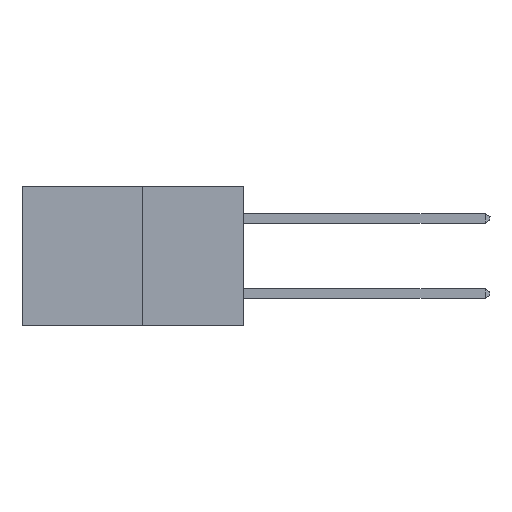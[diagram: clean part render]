
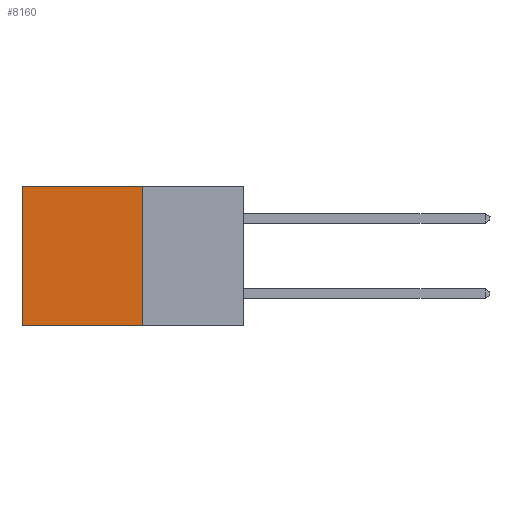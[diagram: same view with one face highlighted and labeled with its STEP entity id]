
A CAD part, left-side view. The second image highlights one B-rep face of the part: STEP entity #8160.
In plain terms, the highlighted planar face has unit normal (-1, 0, 0).
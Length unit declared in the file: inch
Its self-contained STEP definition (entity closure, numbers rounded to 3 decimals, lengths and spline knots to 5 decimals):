
#1149 = EDGE_CURVE ( 'NONE', #7648, #6884, #10491, .T. ) ;
#1304 = FACE_OUTER_BOUND ( 'NONE', #7116, .T. ) ;
#1664 = VERTEX_POINT ( 'NONE', #15203 ) ;
#2497 = VECTOR ( 'NONE', #5993, 39.37008 ) ;
#3135 = ORIENTED_EDGE ( 'NONE', *, *, #1149, .F. ) ;
#3590 = DIRECTION ( 'NONE',  ( 0., 0., -1. ) ) ;
#3797 = CARTESIAN_POINT ( 'NONE',  ( 0.277, 0.27, -0.37 ) ) ;
#4879 = ORIENTED_EDGE ( 'NONE', *, *, #9303, .T. ) ;
#5075 = DIRECTION ( 'NONE',  ( 0., 0., -1. ) ) ;
#5313 = DIRECTION ( 'NONE',  ( 1., 0., 0. ) ) ;
#5993 = DIRECTION ( 'NONE',  ( 0., 1., 0. ) ) ;
#6261 = CARTESIAN_POINT ( 'NONE',  ( 0.277, 0.59, -0.37 ) ) ;
#6416 = AXIS2_PLACEMENT_3D ( 'NONE', #3797, #5313, #15777 ) ;
#6680 = VECTOR ( 'NONE', #3590, 39.37008 ) ;
#6884 = VERTEX_POINT ( 'NONE', #6261 ) ;
#7101 = CARTESIAN_POINT ( 'NONE',  ( 0.277, 0.27, -0.37 ) ) ;
#7116 = EDGE_LOOP ( 'NONE', ( #18130, #3135, #7374, #4879 ) ) ;
#7374 = ORIENTED_EDGE ( 'NONE', *, *, #17259, .F. ) ;
#7406 = EDGE_CURVE ( 'NONE', #9163, #6884, #15392, .T. ) ;
#7648 = VERTEX_POINT ( 'NONE', #7101 ) ;
#8160 = ADVANCED_FACE ( 'NONE', ( #1304 ), #12780, .F. ) ;
#9163 = VERTEX_POINT ( 'NONE', #11904 ) ;
#9303 = EDGE_CURVE ( 'NONE', #1664, #9163, #18601, .T. ) ;
#10491 = LINE ( 'NONE', #16869, #2497 ) ;
#11904 = CARTESIAN_POINT ( 'NONE',  ( 0.277, 0.59, 0. ) ) ;
#12219 = CARTESIAN_POINT ( 'NONE',  ( 0.277, 0.27, 0. ) ) ;
#12780 = PLANE ( 'NONE',  #6416 ) ;
#13712 = DIRECTION ( 'NONE',  ( 0., 1., 0. ) ) ;
#14925 = VECTOR ( 'NONE', #5075, 39.37008 ) ;
#15203 = CARTESIAN_POINT ( 'NONE',  ( 0.277, 0.27, 0. ) ) ;
#15392 = LINE ( 'NONE', #15530, #14925 ) ;
#15530 = CARTESIAN_POINT ( 'NONE',  ( 0.277, 0.59, -0.37 ) ) ;
#15777 = DIRECTION ( 'NONE',  ( 0., 0., -1. ) ) ;
#16869 = CARTESIAN_POINT ( 'NONE',  ( 0.277, 0.27, -0.37 ) ) ;
#17081 = CARTESIAN_POINT ( 'NONE',  ( 0.277, 0.27, -0.37 ) ) ;
#17259 = EDGE_CURVE ( 'NONE', #1664, #7648, #18577, .T. ) ;
#17674 = VECTOR ( 'NONE', #13712, 39.37008 ) ;
#18130 = ORIENTED_EDGE ( 'NONE', *, *, #7406, .T. ) ;
#18577 = LINE ( 'NONE', #17081, #6680 ) ;
#18601 = LINE ( 'NONE', #12219, #17674 ) ;
